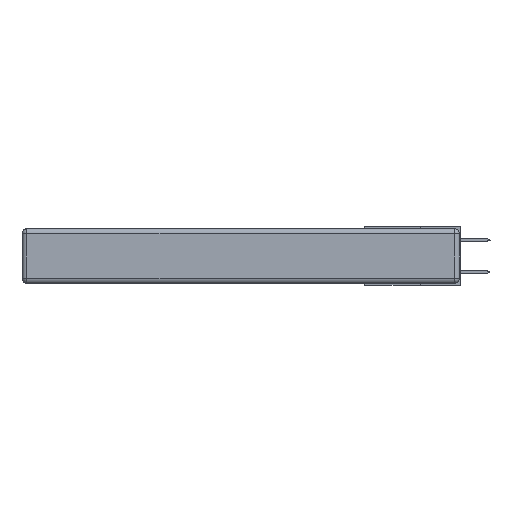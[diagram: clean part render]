
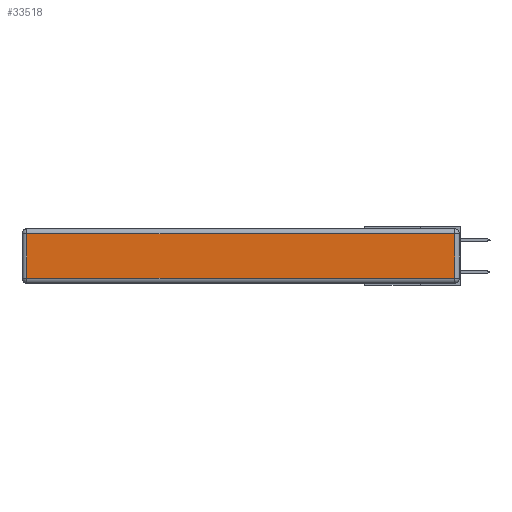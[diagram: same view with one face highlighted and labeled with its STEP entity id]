
A CAD part, left-side view. The second image highlights one B-rep face of the part: STEP entity #33518.
In plain terms, the highlighted planar face has unit normal (-1, 0, 0).
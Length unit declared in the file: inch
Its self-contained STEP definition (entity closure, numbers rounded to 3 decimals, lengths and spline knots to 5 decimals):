
#604 = EDGE_LOOP ( 'NONE', ( #6615, #13043, #16651, #9922 ) ) ;
#1324 = LINE ( 'NONE', #18623, #16049 ) ;
#2077 = VERTEX_POINT ( 'NONE', #10563 ) ;
#2481 = DIRECTION ( 'NONE',  ( 0., 0., 1. ) ) ;
#6247 = CARTESIAN_POINT ( 'NONE',  ( 0., 0.03, -0.313 ) ) ;
#6250 = VECTOR ( 'NONE', #22730, 39.37008 ) ;
#6325 = VERTEX_POINT ( 'NONE', #25774 ) ;
#6615 = ORIENTED_EDGE ( 'NONE', *, *, #8076, .T. ) ;
#7778 = CARTESIAN_POINT ( 'NONE',  ( 0., 0., -0.313 ) ) ;
#8076 = EDGE_CURVE ( 'NONE', #32219, #20454, #33482, .T. ) ;
#9922 = ORIENTED_EDGE ( 'NONE', *, *, #29746, .T. ) ;
#10563 = CARTESIAN_POINT ( 'NONE',  ( 0., 2.72, -0.03 ) ) ;
#11962 = DIRECTION ( 'NONE',  ( -1., 0., 0. ) ) ;
#13043 = ORIENTED_EDGE ( 'NONE', *, *, #30795, .T. ) ;
#15086 = LINE ( 'NONE', #15630, #6250 ) ;
#15630 = CARTESIAN_POINT ( 'NONE',  ( 0., 2.75, -0.03 ) ) ;
#15670 = LINE ( 'NONE', #17497, #24159 ) ;
#16049 = VECTOR ( 'NONE', #2481, 39.37008 ) ;
#16651 = ORIENTED_EDGE ( 'NONE', *, *, #34116, .T. ) ;
#17497 = CARTESIAN_POINT ( 'NONE',  ( 0., 2.72, -0.343 ) ) ;
#18623 = CARTESIAN_POINT ( 'NONE',  ( 0., 0.03, -0.343 ) ) ;
#20357 = DIRECTION ( 'NONE',  ( 0., 0., 1. ) ) ;
#20454 = VERTEX_POINT ( 'NONE', #6247 ) ;
#20558 = CARTESIAN_POINT ( 'NONE',  ( 0., 2.72, -0.313 ) ) ;
#21021 = DIRECTION ( 'NONE',  ( 0., -1., 0. ) ) ;
#22730 = DIRECTION ( 'NONE',  ( 0., 1., 0. ) ) ;
#24159 = VECTOR ( 'NONE', #25513, 39.37008 ) ;
#25513 = DIRECTION ( 'NONE',  ( 0., 0., -1. ) ) ;
#25745 = CARTESIAN_POINT ( 'NONE',  ( 0., 0., -0.343 ) ) ;
#25774 = CARTESIAN_POINT ( 'NONE',  ( 0., 0.03, -0.03 ) ) ;
#28464 = PLANE ( 'NONE',  #34350 ) ;
#29042 = FACE_OUTER_BOUND ( 'NONE', #604, .T. ) ;
#29305 = VECTOR ( 'NONE', #21021, 39.37008 ) ;
#29746 = EDGE_CURVE ( 'NONE', #2077, #32219, #15670, .T. ) ;
#30795 = EDGE_CURVE ( 'NONE', #20454, #6325, #1324, .T. ) ;
#32219 = VERTEX_POINT ( 'NONE', #20558 ) ;
#33482 = LINE ( 'NONE', #7778, #29305 ) ;
#33518 = ADVANCED_FACE ( 'NONE', ( #29042 ), #28464, .T. ) ;
#34116 = EDGE_CURVE ( 'NONE', #6325, #2077, #15086, .T. ) ;
#34350 = AXIS2_PLACEMENT_3D ( 'NONE', #25745, #11962, #20357 ) ;
